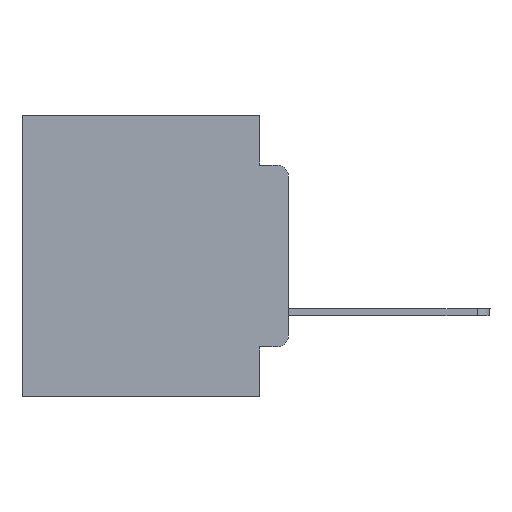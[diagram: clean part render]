
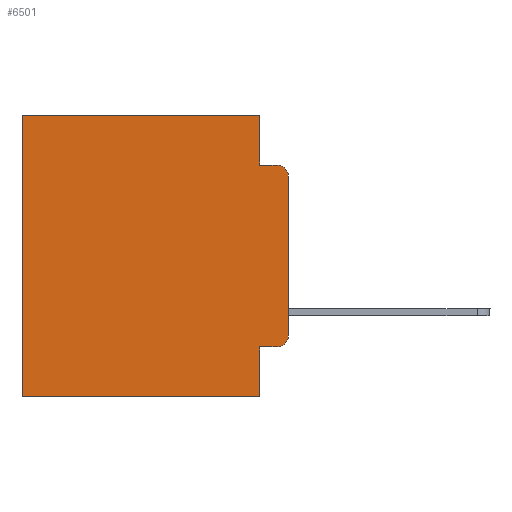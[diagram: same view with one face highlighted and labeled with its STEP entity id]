
A CAD part, left-side view. The second image highlights one B-rep face of the part: STEP entity #6501.
In plain terms, the highlighted planar face has unit normal (-1, 0, 0).
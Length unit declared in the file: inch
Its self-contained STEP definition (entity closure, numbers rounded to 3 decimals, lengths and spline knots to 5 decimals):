
#304 = CARTESIAN_POINT ( 'NONE',  ( 0.298, 0.02, -0.4115 ) ) ;
#2264 = AXIS2_PLACEMENT_3D ( 'NONE', #5813, #22802, #26887 ) ;
#2482 = DIRECTION ( 'NONE',  ( 0., 0., -1. ) ) ;
#2614 = VECTOR ( 'NONE', #3206, 39.37008 ) ;
#2623 = ORIENTED_EDGE ( 'NONE', *, *, #16588, .F. ) ;
#2781 = LINE ( 'NONE', #19515, #14600 ) ;
#2872 = CIRCLE ( 'NONE', #22883, 0.02 ) ;
#3206 = DIRECTION ( 'NONE',  ( 0., 0., -1. ) ) ;
#3364 = ORIENTED_EDGE ( 'NONE', *, *, #23816, .T. ) ;
#3988 = DIRECTION ( 'NONE',  ( -1., 0., 0. ) ) ;
#4132 = EDGE_LOOP ( 'NONE', ( #13010, #5420, #2623, #20729, #3364, #14228, #15795, #6012, #13741, #10064 ) ) ;
#4463 = EDGE_CURVE ( 'NONE', #18052, #23072, #2872, .T. ) ;
#4718 = FACE_OUTER_BOUND ( 'NONE', #4132, .T. ) ;
#5259 = DIRECTION ( 'NONE',  ( 0., 0., -1. ) ) ;
#5420 = ORIENTED_EDGE ( 'NONE', *, *, #4463, .T. ) ;
#5660 = CARTESIAN_POINT ( 'NONE',  ( 0.298, 0.051, -0.4115 ) ) ;
#5813 = CARTESIAN_POINT ( 'NONE',  ( 0.298, 0.02, -0.3915 ) ) ;
#6012 = ORIENTED_EDGE ( 'NONE', *, *, #16495, .F. ) ;
#6201 = VERTEX_POINT ( 'NONE', #16733 ) ;
#6397 = CARTESIAN_POINT ( 'NONE',  ( 0.298, 0., 0. ) ) ;
#6501 = ADVANCED_FACE ( 'NONE', ( #4718 ), #13035, .F. ) ;
#6542 = VERTEX_POINT ( 'NONE', #25953 ) ;
#7013 = VERTEX_POINT ( 'NONE', #304 ) ;
#7033 = LINE ( 'NONE', #15330, #2614 ) ;
#7647 = EDGE_CURVE ( 'NONE', #19243, #7013, #9220, .T. ) ;
#7713 = CARTESIAN_POINT ( 'NONE',  ( 0.298, 0.051, 0. ) ) ;
#8692 = LINE ( 'NONE', #6397, #19710 ) ;
#8827 = EDGE_CURVE ( 'NONE', #9017, #6542, #19678, .T. ) ;
#8938 = DIRECTION ( 'NONE',  ( 0., 0., -1. ) ) ;
#9017 = VERTEX_POINT ( 'NONE', #7713 ) ;
#9220 = LINE ( 'NONE', #17094, #15105 ) ;
#10064 = ORIENTED_EDGE ( 'NONE', *, *, #22063, .T. ) ;
#10685 = VECTOR ( 'NONE', #8938, 39.37008 ) ;
#10802 = CARTESIAN_POINT ( 'NONE',  ( 0.298, 0.02, -0.1085 ) ) ;
#10807 = CARTESIAN_POINT ( 'NONE',  ( 0.298, 0.051, -0.5 ) ) ;
#11007 = CARTESIAN_POINT ( 'NONE',  ( 0.298, 0.051, 0. ) ) ;
#11172 = EDGE_CURVE ( 'NONE', #18052, #16316, #7033, .T. ) ;
#11333 = CARTESIAN_POINT ( 'NONE',  ( 0.298, 0.02, -0.0885 ) ) ;
#11514 = LINE ( 'NONE', #17879, #24596 ) ;
#11712 = CARTESIAN_POINT ( 'NONE',  ( 0.298, 0., -0.5 ) ) ;
#11827 = AXIS2_PLACEMENT_3D ( 'NONE', #21311, #21712, #17761 ) ;
#12502 = LINE ( 'NONE', #14522, #10685 ) ;
#12544 = VECTOR ( 'NONE', #13176, 39.37008 ) ;
#13010 = ORIENTED_EDGE ( 'NONE', *, *, #11172, .F. ) ;
#13035 = PLANE ( 'NONE',  #11827 ) ;
#13176 = DIRECTION ( 'NONE',  ( 0., 0., -1. ) ) ;
#13323 = VERTEX_POINT ( 'NONE', #10807 ) ;
#13741 = ORIENTED_EDGE ( 'NONE', *, *, #7647, .T. ) ;
#14228 = ORIENTED_EDGE ( 'NONE', *, *, #25752, .T. ) ;
#14522 = CARTESIAN_POINT ( 'NONE',  ( 0.298, 0.051, 0. ) ) ;
#14600 = VECTOR ( 'NONE', #21833, 39.37008 ) ;
#15076 = DIRECTION ( 'NONE',  ( 0., -1., 0. ) ) ;
#15105 = VECTOR ( 'NONE', #15076, 39.37008 ) ;
#15330 = CARTESIAN_POINT ( 'NONE',  ( 0.298, 0., 0. ) ) ;
#15512 = LINE ( 'NONE', #11712, #20565 ) ;
#15622 = CARTESIAN_POINT ( 'NONE',  ( 0.298, 0., -0.1085 ) ) ;
#15795 = ORIENTED_EDGE ( 'NONE', *, *, #23483, .F. ) ;
#15932 = VERTEX_POINT ( 'NONE', #26306 ) ;
#16316 = VERTEX_POINT ( 'NONE', #17535 ) ;
#16495 = EDGE_CURVE ( 'NONE', #19243, #13323, #12502, .T. ) ;
#16588 = EDGE_CURVE ( 'NONE', #6542, #23072, #2781, .T. ) ;
#16733 = CARTESIAN_POINT ( 'NONE',  ( 0.298, 0.473, 0. ) ) ;
#17094 = CARTESIAN_POINT ( 'NONE',  ( 0.298, 0.051, -0.4115 ) ) ;
#17535 = CARTESIAN_POINT ( 'NONE',  ( 0.298, 0., -0.3915 ) ) ;
#17761 = DIRECTION ( 'NONE',  ( 0., 0., -1. ) ) ;
#17879 = CARTESIAN_POINT ( 'NONE',  ( 0.298, 0.473, 0. ) ) ;
#18052 = VERTEX_POINT ( 'NONE', #15622 ) ;
#19243 = VERTEX_POINT ( 'NONE', #5660 ) ;
#19515 = CARTESIAN_POINT ( 'NONE',  ( 0.298, 0.051, -0.0885 ) ) ;
#19678 = LINE ( 'NONE', #11007, #12544 ) ;
#19710 = VECTOR ( 'NONE', #22985, 39.37008 ) ;
#20565 = VECTOR ( 'NONE', #21899, 39.37008 ) ;
#20729 = ORIENTED_EDGE ( 'NONE', *, *, #8827, .F. ) ;
#21311 = CARTESIAN_POINT ( 'NONE',  ( 0.298, 0., 0. ) ) ;
#21712 = DIRECTION ( 'NONE',  ( 1., 0., 0. ) ) ;
#21833 = DIRECTION ( 'NONE',  ( 0., -1., 0. ) ) ;
#21899 = DIRECTION ( 'NONE',  ( 0., 1., 0. ) ) ;
#22063 = EDGE_CURVE ( 'NONE', #7013, #16316, #26600, .T. ) ;
#22802 = DIRECTION ( 'NONE',  ( -1., 0., 0. ) ) ;
#22883 = AXIS2_PLACEMENT_3D ( 'NONE', #10802, #3988, #2482 ) ;
#22985 = DIRECTION ( 'NONE',  ( 0., 1., 0. ) ) ;
#23072 = VERTEX_POINT ( 'NONE', #11333 ) ;
#23483 = EDGE_CURVE ( 'NONE', #13323, #15932, #15512, .T. ) ;
#23816 = EDGE_CURVE ( 'NONE', #9017, #6201, #8692, .T. ) ;
#24596 = VECTOR ( 'NONE', #5259, 39.37008 ) ;
#25752 = EDGE_CURVE ( 'NONE', #6201, #15932, #11514, .T. ) ;
#25953 = CARTESIAN_POINT ( 'NONE',  ( 0.298, 0.051, -0.0885 ) ) ;
#26306 = CARTESIAN_POINT ( 'NONE',  ( 0.298, 0.473, -0.5 ) ) ;
#26600 = CIRCLE ( 'NONE', #2264, 0.02 ) ;
#26887 = DIRECTION ( 'NONE',  ( 0., 0., -1. ) ) ;
